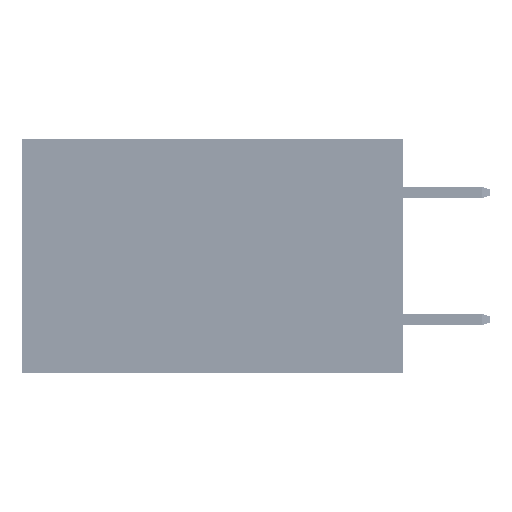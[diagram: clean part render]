
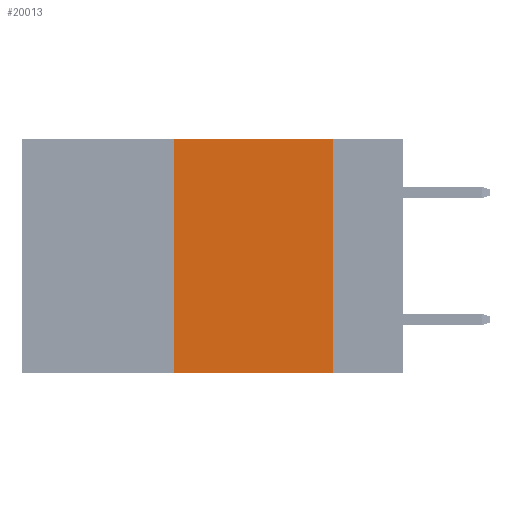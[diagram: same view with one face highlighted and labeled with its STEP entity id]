
A CAD part, left-side view. The second image highlights one B-rep face of the part: STEP entity #20013.
In plain terms, the highlighted planar face has unit normal (-1, 0, 0).
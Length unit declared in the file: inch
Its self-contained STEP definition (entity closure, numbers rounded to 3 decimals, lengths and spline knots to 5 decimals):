
#1680 = DIRECTION ( 'NONE',  ( 1., 0., 0. ) ) ;
#2652 = CARTESIAN_POINT ( 'NONE',  ( 0., 0.11, 0. ) ) ;
#4713 = ORIENTED_EDGE ( 'NONE', *, *, #31070, .F. ) ;
#5473 = VERTEX_POINT ( 'NONE', #48963 ) ;
#5790 = CARTESIAN_POINT ( 'NONE',  ( 0., 0.6, -0.37 ) ) ;
#5951 = LINE ( 'NONE', #42700, #44218 ) ;
#8824 = CARTESIAN_POINT ( 'NONE',  ( 0., 0.36, 0. ) ) ;
#9036 = ORIENTED_EDGE ( 'NONE', *, *, #34053, .F. ) ;
#9037 = VECTOR ( 'NONE', #21486, 39.37008 ) ;
#9788 = LINE ( 'NONE', #5790, #9037 ) ;
#10756 = DIRECTION ( 'NONE',  ( 0., 0., -1. ) ) ;
#13483 = FACE_OUTER_BOUND ( 'NONE', #37728, .T. ) ;
#16747 = LINE ( 'NONE', #32990, #42538 ) ;
#19573 = EDGE_CURVE ( 'NONE', #5473, #51479, #9788, .T. ) ;
#20013 = ADVANCED_FACE ( 'NONE', ( #13483 ), #37140, .F. ) ;
#21486 = DIRECTION ( 'NONE',  ( 0., -1., 0. ) ) ;
#24881 = VECTOR ( 'NONE', #47873, 39.37008 ) ;
#26126 = ORIENTED_EDGE ( 'NONE', *, *, #19573, .T. ) ;
#29453 = AXIS2_PLACEMENT_3D ( 'NONE', #49705, #1680, #33926 ) ;
#30081 = CARTESIAN_POINT ( 'NONE',  ( 0., 0.36, 0. ) ) ;
#31070 = EDGE_CURVE ( 'NONE', #5473, #48082, #51913, .T. ) ;
#32990 = CARTESIAN_POINT ( 'NONE',  ( 0., 0.6, 0. ) ) ;
#33926 = DIRECTION ( 'NONE',  ( 0., 0., -1. ) ) ;
#34053 = EDGE_CURVE ( 'NONE', #39914, #51479, #5951, .T. ) ;
#36150 = EDGE_CURVE ( 'NONE', #48082, #39914, #16747, .T. ) ;
#37140 = PLANE ( 'NONE',  #29453 ) ;
#37728 = EDGE_LOOP ( 'NONE', ( #9036, #42011, #4713, #26126 ) ) ;
#39775 = CARTESIAN_POINT ( 'NONE',  ( 0., 0.11, -0.37 ) ) ;
#39914 = VERTEX_POINT ( 'NONE', #2652 ) ;
#42011 = ORIENTED_EDGE ( 'NONE', *, *, #36150, .F. ) ;
#42538 = VECTOR ( 'NONE', #49257, 39.37008 ) ;
#42700 = CARTESIAN_POINT ( 'NONE',  ( 0., 0.11, 0. ) ) ;
#44218 = VECTOR ( 'NONE', #10756, 39.37008 ) ;
#47873 = DIRECTION ( 'NONE',  ( 0., 0., 1. ) ) ;
#48082 = VERTEX_POINT ( 'NONE', #8824 ) ;
#48963 = CARTESIAN_POINT ( 'NONE',  ( 0., 0.36, -0.37 ) ) ;
#49257 = DIRECTION ( 'NONE',  ( 0., -1., 0. ) ) ;
#49705 = CARTESIAN_POINT ( 'NONE',  ( 0., 0.6, 0. ) ) ;
#51479 = VERTEX_POINT ( 'NONE', #39775 ) ;
#51913 = LINE ( 'NONE', #30081, #24881 ) ;
